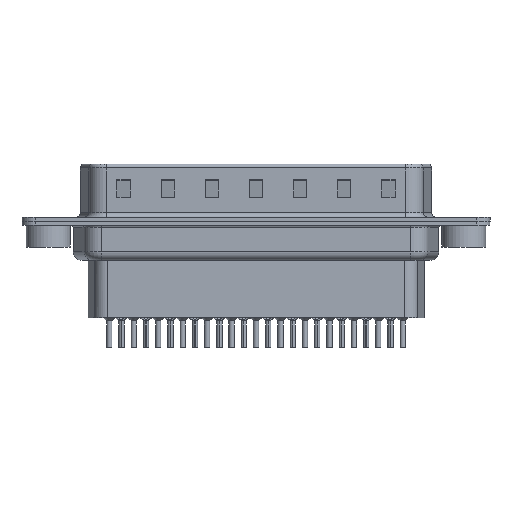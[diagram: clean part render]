
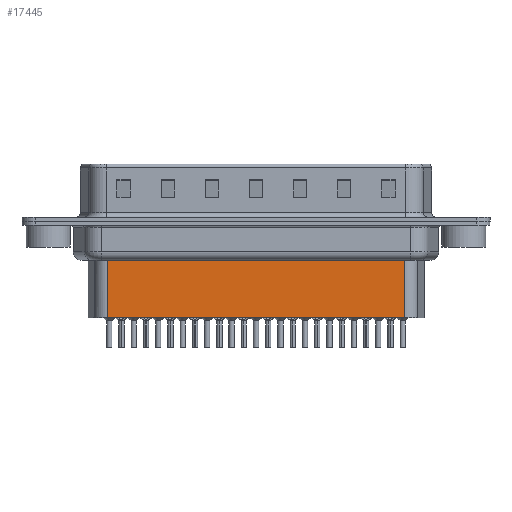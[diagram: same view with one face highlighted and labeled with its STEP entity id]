
A CAD part, front view. The second image highlights one B-rep face of the part: STEP entity #17445.
In plain terms, the highlighted planar face has unit normal (0, -1, 0).
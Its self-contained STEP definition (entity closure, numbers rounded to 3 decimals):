
#165 = PLANE ( 'NONE',  #23687 ) ;
#1536 = VERTEX_POINT ( 'NONE', #1843 ) ;
#1843 = CARTESIAN_POINT ( 'NONE',  ( 40.344, -3.5, -10.95 ) ) ;
#2282 = EDGE_CURVE ( 'NONE', #16406, #17332, #17488, .T. ) ;
#3973 = DIRECTION ( 'NONE',  ( 0., -1., 0. ) ) ;
#4351 = DIRECTION ( 'NONE',  ( 1., 0., 0. ) ) ;
#4943 = DIRECTION ( 'NONE',  ( -1., 0., 0. ) ) ;
#6464 = LINE ( 'NONE', #15617, #7767 ) ;
#7735 = EDGE_LOOP ( 'NONE', ( #18040, #10666, #13373, #24598 ) ) ;
#7767 = VECTOR ( 'NONE', #15852, 1000. ) ;
#9392 = CARTESIAN_POINT ( 'NONE',  ( 40.344, -3.5, -3.1 ) ) ;
#9461 = VECTOR ( 'NONE', #13080, 1000. ) ;
#10246 = EDGE_CURVE ( 'NONE', #1536, #17332, #17116, .T. ) ;
#10666 = ORIENTED_EDGE ( 'NONE', *, *, #12811, .T. ) ;
#10979 = CARTESIAN_POINT ( 'NONE',  ( 40.344, -3.5, -4.097 ) ) ;
#11344 = EDGE_CURVE ( 'NONE', #17376, #1536, #20835, .T. ) ;
#12811 = EDGE_CURVE ( 'NONE', #17376, #16406, #6464, .T. ) ;
#13005 = CARTESIAN_POINT ( 'NONE',  ( 6.706, -3.5, -10.95 ) ) ;
#13080 = DIRECTION ( 'NONE',  ( 0., 0., -1. ) ) ;
#13373 = ORIENTED_EDGE ( 'NONE', *, *, #2282, .T. ) ;
#14334 = VECTOR ( 'NONE', #23214, 1000. ) ;
#15617 = CARTESIAN_POINT ( 'NONE',  ( 6.459, -3.5, -4.097 ) ) ;
#15852 = DIRECTION ( 'NONE',  ( -1., 0., 0. ) ) ;
#16406 = VERTEX_POINT ( 'NONE', #24739 ) ;
#17116 = LINE ( 'NONE', #22327, #24399 ) ;
#17332 = VERTEX_POINT ( 'NONE', #13005 ) ;
#17376 = VERTEX_POINT ( 'NONE', #10979 ) ;
#17445 = ADVANCED_FACE ( 'NONE', ( #23415 ), #165, .T. ) ;
#17488 = LINE ( 'NONE', #18822, #14334 ) ;
#18040 = ORIENTED_EDGE ( 'NONE', *, *, #11344, .F. ) ;
#18822 = CARTESIAN_POINT ( 'NONE',  ( 6.706, -3.5, -3.1 ) ) ;
#19723 = CARTESIAN_POINT ( 'NONE',  ( 6.706, -3.5, -3.1 ) ) ;
#20835 = LINE ( 'NONE', #9392, #9461 ) ;
#22327 = CARTESIAN_POINT ( 'NONE',  ( 6.706, -3.5, -10.95 ) ) ;
#23214 = DIRECTION ( 'NONE',  ( 0., 0., -1. ) ) ;
#23415 = FACE_OUTER_BOUND ( 'NONE', #7735, .T. ) ;
#23687 = AXIS2_PLACEMENT_3D ( 'NONE', #19723, #3973, #4351 ) ;
#24399 = VECTOR ( 'NONE', #4943, 1000. ) ;
#24598 = ORIENTED_EDGE ( 'NONE', *, *, #10246, .F. ) ;
#24739 = CARTESIAN_POINT ( 'NONE',  ( 6.706, -3.5, -4.097 ) ) ;
